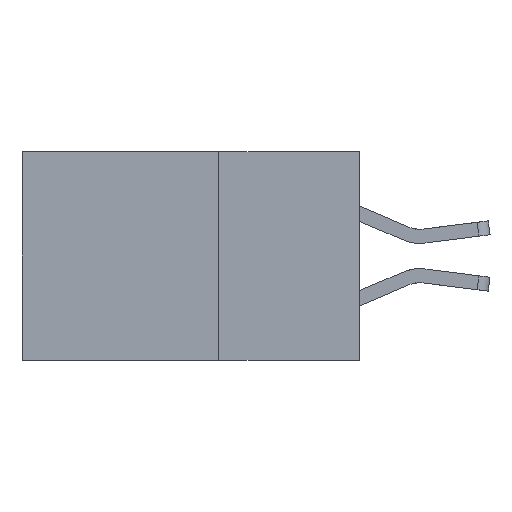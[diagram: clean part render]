
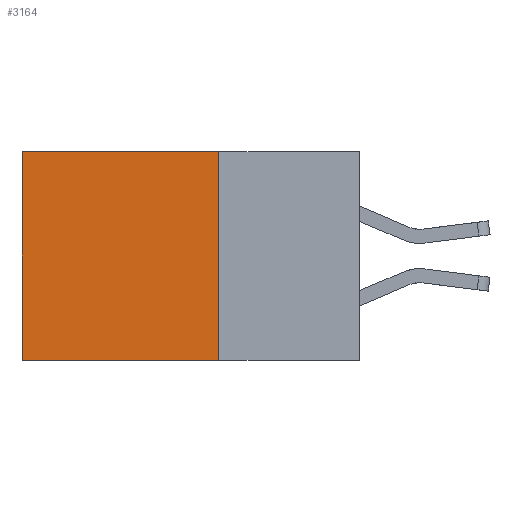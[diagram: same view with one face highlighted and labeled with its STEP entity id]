
A CAD part, left-side view. The second image highlights one B-rep face of the part: STEP entity #3164.
In plain terms, the highlighted planar face has unit normal (-1, 0, 0).
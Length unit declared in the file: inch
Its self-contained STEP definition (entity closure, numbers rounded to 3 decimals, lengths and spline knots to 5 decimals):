
#19 = FACE_OUTER_BOUND ( 'NONE', #3078, .T. ) ;
#494 = VERTEX_POINT ( 'NONE', #2400 ) ;
#996 = ORIENTED_EDGE ( 'NONE', *, *, #4998, .F. ) ;
#1062 = DIRECTION ( 'NONE',  ( 0., 1., 0. ) ) ;
#1539 = DIRECTION ( 'NONE',  ( 1., 0., 0. ) ) ;
#2199 = VECTOR ( 'NONE', #4392, 39.37008 ) ;
#2400 = CARTESIAN_POINT ( 'NONE',  ( 0.2875, 0.25, 0. ) ) ;
#2882 = LINE ( 'NONE', #10074, #2199 ) ;
#3078 = EDGE_LOOP ( 'NONE', ( #9344, #7165, #996, #3858 ) ) ;
#3098 = CARTESIAN_POINT ( 'NONE',  ( 0.2875, 0.6, -0.37 ) ) ;
#3159 = VECTOR ( 'NONE', #5404, 39.37008 ) ;
#3164 = ADVANCED_FACE ( 'NONE', ( #19 ), #3834, .F. ) ;
#3297 = EDGE_CURVE ( 'NONE', #9163, #4850, #9772, .T. ) ;
#3306 = LINE ( 'NONE', #7368, #3687 ) ;
#3467 = CARTESIAN_POINT ( 'NONE',  ( 0.2875, 0.25, -0.37 ) ) ;
#3687 = VECTOR ( 'NONE', #4185, 39.37008 ) ;
#3714 = AXIS2_PLACEMENT_3D ( 'NONE', #9411, #1539, #4775 ) ;
#3788 = LINE ( 'NONE', #7850, #3159 ) ;
#3834 = PLANE ( 'NONE',  #3714 ) ;
#3858 = ORIENTED_EDGE ( 'NONE', *, *, #8771, .T. ) ;
#4130 = VECTOR ( 'NONE', #1062, 39.37008 ) ;
#4185 = DIRECTION ( 'NONE',  ( 0., 0., -1. ) ) ;
#4392 = DIRECTION ( 'NONE',  ( 0., 0., -1. ) ) ;
#4775 = DIRECTION ( 'NONE',  ( 0., 0., -1. ) ) ;
#4850 = VERTEX_POINT ( 'NONE', #3098 ) ;
#4998 = EDGE_CURVE ( 'NONE', #494, #9163, #3306, .T. ) ;
#5141 = EDGE_CURVE ( 'NONE', #9559, #4850, #2882, .T. ) ;
#5404 = DIRECTION ( 'NONE',  ( 0., 1., 0. ) ) ;
#7165 = ORIENTED_EDGE ( 'NONE', *, *, #3297, .F. ) ;
#7368 = CARTESIAN_POINT ( 'NONE',  ( 0.2875, 0.25, 0. ) ) ;
#7376 = CARTESIAN_POINT ( 'NONE',  ( 0.2875, 0.25, -0.37 ) ) ;
#7850 = CARTESIAN_POINT ( 'NONE',  ( 0.2875, 0.25, 0. ) ) ;
#8524 = CARTESIAN_POINT ( 'NONE',  ( 0.2875, 0.6, 0. ) ) ;
#8771 = EDGE_CURVE ( 'NONE', #494, #9559, #3788, .T. ) ;
#9163 = VERTEX_POINT ( 'NONE', #3467 ) ;
#9344 = ORIENTED_EDGE ( 'NONE', *, *, #5141, .T. ) ;
#9411 = CARTESIAN_POINT ( 'NONE',  ( 0.2875, 0.25, 0. ) ) ;
#9559 = VERTEX_POINT ( 'NONE', #8524 ) ;
#9772 = LINE ( 'NONE', #7376, #4130 ) ;
#10074 = CARTESIAN_POINT ( 'NONE',  ( 0.2875, 0.6, 0. ) ) ;
